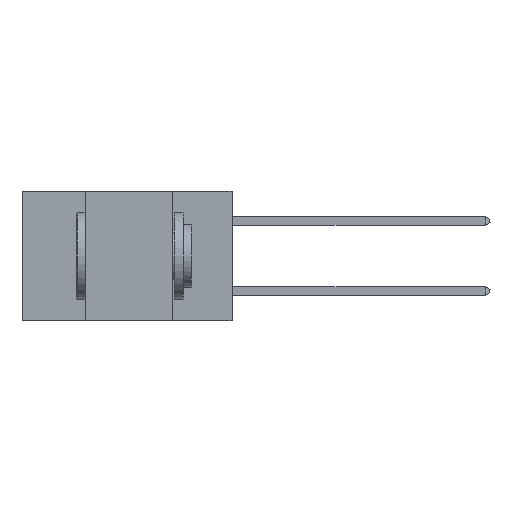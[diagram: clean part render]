
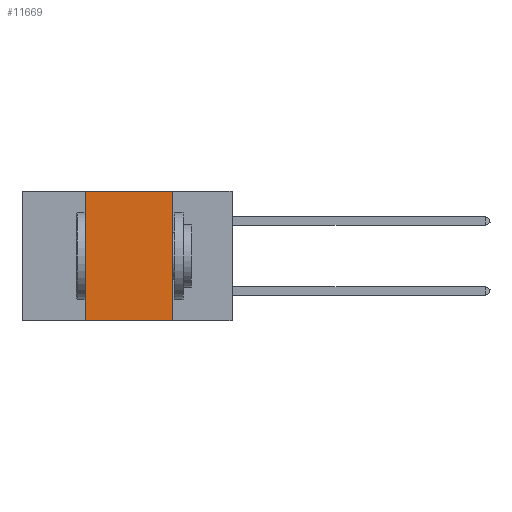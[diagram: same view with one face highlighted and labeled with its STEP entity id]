
A CAD part, left-side view. The second image highlights one B-rep face of the part: STEP entity #11669.
In plain terms, the highlighted planar face has unit normal (-1, 0, 0).
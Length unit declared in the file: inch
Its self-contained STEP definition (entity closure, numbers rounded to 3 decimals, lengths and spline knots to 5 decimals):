
#30 = EDGE_CURVE ( 'NONE', #31874, #22781, #13749, .T. ) ;
#299 = CARTESIAN_POINT ( 'NONE',  ( 0., 0.17, -0.37 ) ) ;
#1234 = ORIENTED_EDGE ( 'NONE', *, *, #10307, .T. ) ;
#1694 = EDGE_CURVE ( 'NONE', #23553, #31874, #5452, .T. ) ;
#2450 = DIRECTION ( 'NONE',  ( 0., 0., -1. ) ) ;
#2688 = CARTESIAN_POINT ( 'NONE',  ( 0., 0.42, -0.37 ) ) ;
#2831 = AXIS2_PLACEMENT_3D ( 'NONE', #16774, #19542, #2450 ) ;
#3488 = CARTESIAN_POINT ( 'NONE',  ( 0., 0.17, 0. ) ) ;
#5452 = LINE ( 'NONE', #32469, #27749 ) ;
#6255 = ORIENTED_EDGE ( 'NONE', *, *, #30, .F. ) ;
#10307 = EDGE_CURVE ( 'NONE', #23553, #30839, #18059, .T. ) ;
#11406 = DIRECTION ( 'NONE',  ( 0., -1., 0. ) ) ;
#11588 = FACE_OUTER_BOUND ( 'NONE', #33724, .T. ) ;
#11669 = ADVANCED_FACE ( 'NONE', ( #11588 ), #13995, .F. ) ;
#12026 = CARTESIAN_POINT ( 'NONE',  ( 0., 0.6, 0. ) ) ;
#13399 = DIRECTION ( 'NONE',  ( 0., 0., 1. ) ) ;
#13749 = LINE ( 'NONE', #12026, #21052 ) ;
#13995 = PLANE ( 'NONE',  #2831 ) ;
#15174 = DIRECTION ( 'NONE',  ( 0., 0., -1. ) ) ;
#15722 = ORIENTED_EDGE ( 'NONE', *, *, #1694, .F. ) ;
#16128 = ORIENTED_EDGE ( 'NONE', *, *, #33952, .F. ) ;
#16650 = CARTESIAN_POINT ( 'NONE',  ( 0., 0.42, 0. ) ) ;
#16774 = CARTESIAN_POINT ( 'NONE',  ( 0., 0.6, 0. ) ) ;
#18059 = LINE ( 'NONE', #29320, #30819 ) ;
#19542 = DIRECTION ( 'NONE',  ( 1., 0., 0. ) ) ;
#21052 = VECTOR ( 'NONE', #11406, 39.37008 ) ;
#22781 = VERTEX_POINT ( 'NONE', #3488 ) ;
#23553 = VERTEX_POINT ( 'NONE', #2688 ) ;
#24031 = LINE ( 'NONE', #31508, #32933 ) ;
#27749 = VECTOR ( 'NONE', #13399, 39.37008 ) ;
#29320 = CARTESIAN_POINT ( 'NONE',  ( 0., 0.6, -0.37 ) ) ;
#30819 = VECTOR ( 'NONE', #34623, 39.37008 ) ;
#30839 = VERTEX_POINT ( 'NONE', #299 ) ;
#31508 = CARTESIAN_POINT ( 'NONE',  ( 0., 0.17, 0. ) ) ;
#31874 = VERTEX_POINT ( 'NONE', #16650 ) ;
#32469 = CARTESIAN_POINT ( 'NONE',  ( 0., 0.42, 0. ) ) ;
#32933 = VECTOR ( 'NONE', #15174, 39.37008 ) ;
#33724 = EDGE_LOOP ( 'NONE', ( #16128, #6255, #15722, #1234 ) ) ;
#33952 = EDGE_CURVE ( 'NONE', #22781, #30839, #24031, .T. ) ;
#34623 = DIRECTION ( 'NONE',  ( 0., -1., 0. ) ) ;
